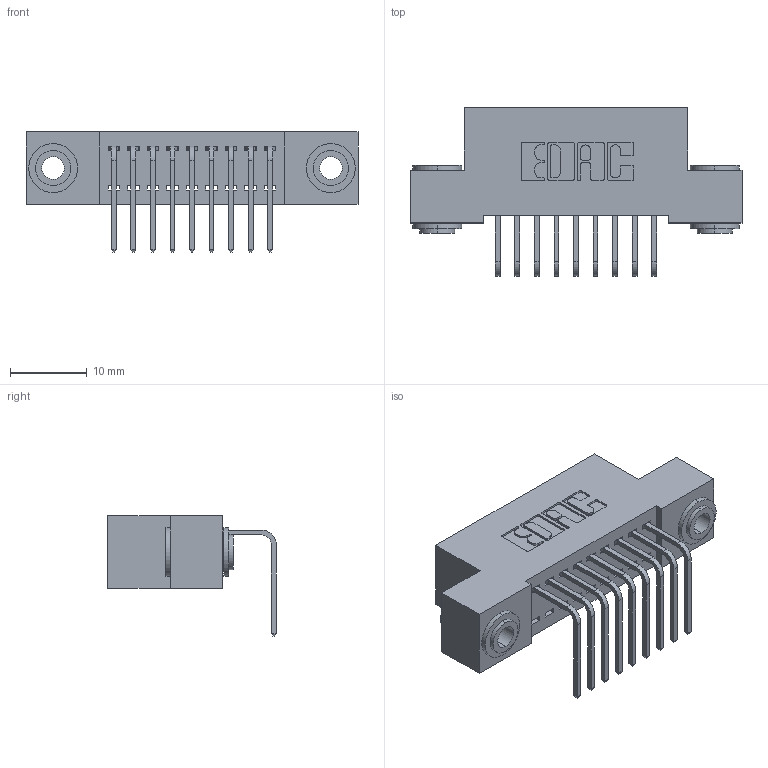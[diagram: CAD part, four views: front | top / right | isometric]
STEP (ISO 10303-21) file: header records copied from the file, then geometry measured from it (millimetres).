
FILE_DESCRIPTION (( 'STEP AP203' ), '1' );
FILE_NAME ('392-009-558-103.STEP', '2018-08-14T19:57:34', ( '' ), ( '' ), 'SwSTEP 2.0', 'SolidWorks 2016', '' );
FILE_SCHEMA (( 'CONFIG_CONTROL_DESIGN' ));
Length unit declared in the file: inch
Products named in the file (4): 345-292-001_558 Tail - 2; 342-250-002_345-250-002-102; 392-009-558-103; 342 Part_.156 TH
Assembly tree (12 placements, depth 2):
  392-009-558-103
    342 Part_.156 TH
    345-292-001_558 Tail - 2  x9
    342-250-002_345-250-002-102  x2
Bounding box: 43.18 x 21.91 x 15.62 mm (x, y, z)
Volume: 3717.3 mm3; surface area: 5239 mm2
Topology: 12 solids, 12 shells, 688 faces, 2013 edges, 1326 vertices
Faces by surface type: plane 472, cylinder 208, cone 8
Entity records: 10372 total; most frequent: CARTESIAN_POINT 1772, ORIENTED_EDGE 1710, DIRECTION 1595, EDGE_CURVE 855, VECTOR 703, LINE 703, VERTEX_POINT 566, AXIS2_PLACEMENT_3D 446
